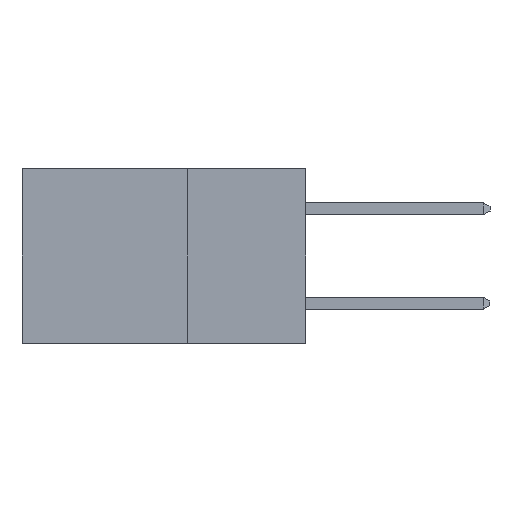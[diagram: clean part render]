
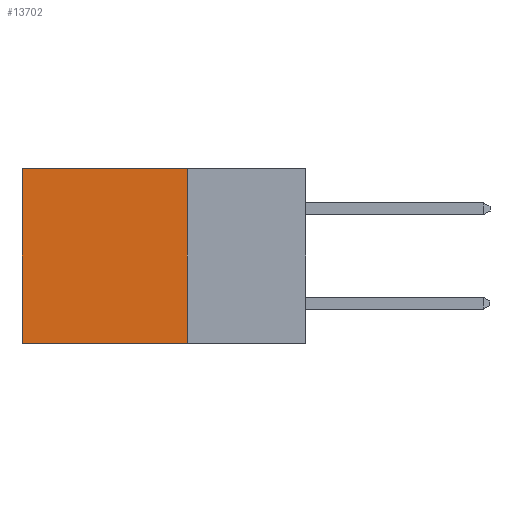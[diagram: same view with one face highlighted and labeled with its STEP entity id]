
A CAD part, left-side view. The second image highlights one B-rep face of the part: STEP entity #13702.
In plain terms, the highlighted planar face has unit normal (-1, 0, 0).
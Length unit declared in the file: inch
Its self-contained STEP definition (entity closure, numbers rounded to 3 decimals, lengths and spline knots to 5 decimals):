
#294 = VERTEX_POINT ( 'NONE', #9446 ) ;
#380 = DIRECTION ( 'NONE',  ( 1., 0., 0. ) ) ;
#1193 = EDGE_LOOP ( 'NONE', ( #5624, #12774, #12250, #18803 ) ) ;
#3577 = DIRECTION ( 'NONE',  ( 0., 1., 0. ) ) ;
#5527 = LINE ( 'NONE', #20162, #17577 ) ;
#5624 = ORIENTED_EDGE ( 'NONE', *, *, #9197, .T. ) ;
#7064 = VERTEX_POINT ( 'NONE', #7242 ) ;
#7242 = CARTESIAN_POINT ( 'NONE',  ( 0.298, 0.25, -0.37 ) ) ;
#7821 = CARTESIAN_POINT ( 'NONE',  ( 0.298, 0.6, 0. ) ) ;
#7977 = VECTOR ( 'NONE', #3577, 39.37008 ) ;
#8087 = LINE ( 'NONE', #19414, #19982 ) ;
#8811 = AXIS2_PLACEMENT_3D ( 'NONE', #9799, #380, #11399 ) ;
#9197 = EDGE_CURVE ( 'NONE', #12243, #294, #19076, .T. ) ;
#9329 = DIRECTION ( 'NONE',  ( 0., 0., -1. ) ) ;
#9446 = CARTESIAN_POINT ( 'NONE',  ( 0.298, 0.6, -0.37 ) ) ;
#9799 = CARTESIAN_POINT ( 'NONE',  ( 0.298, 0.25, 0. ) ) ;
#9859 = CARTESIAN_POINT ( 'NONE',  ( 0.298, 0.25, 0. ) ) ;
#10257 = EDGE_CURVE ( 'NONE', #7064, #294, #8087, .T. ) ;
#10807 = VECTOR ( 'NONE', #15410, 39.37008 ) ;
#11399 = DIRECTION ( 'NONE',  ( 0., 0., -1. ) ) ;
#12167 = LINE ( 'NONE', #9859, #7977 ) ;
#12223 = EDGE_CURVE ( 'NONE', #13657, #7064, #5527, .T. ) ;
#12243 = VERTEX_POINT ( 'NONE', #7821 ) ;
#12250 = ORIENTED_EDGE ( 'NONE', *, *, #12223, .F. ) ;
#12774 = ORIENTED_EDGE ( 'NONE', *, *, #10257, .F. ) ;
#13657 = VERTEX_POINT ( 'NONE', #17504 ) ;
#13702 = ADVANCED_FACE ( 'NONE', ( #19154 ), #17623, .F. ) ;
#15410 = DIRECTION ( 'NONE',  ( 0., 0., -1. ) ) ;
#17504 = CARTESIAN_POINT ( 'NONE',  ( 0.298, 0.25, 0. ) ) ;
#17577 = VECTOR ( 'NONE', #9329, 39.37008 ) ;
#17623 = PLANE ( 'NONE',  #8811 ) ;
#18763 = CARTESIAN_POINT ( 'NONE',  ( 0.298, 0.6, 0. ) ) ;
#18803 = ORIENTED_EDGE ( 'NONE', *, *, #19197, .T. ) ;
#19076 = LINE ( 'NONE', #18763, #10807 ) ;
#19154 = FACE_OUTER_BOUND ( 'NONE', #1193, .T. ) ;
#19197 = EDGE_CURVE ( 'NONE', #13657, #12243, #12167, .T. ) ;
#19414 = CARTESIAN_POINT ( 'NONE',  ( 0.298, 0.25, -0.37 ) ) ;
#19481 = DIRECTION ( 'NONE',  ( 0., 1., 0. ) ) ;
#19982 = VECTOR ( 'NONE', #19481, 39.37008 ) ;
#20162 = CARTESIAN_POINT ( 'NONE',  ( 0.298, 0.25, 0. ) ) ;
